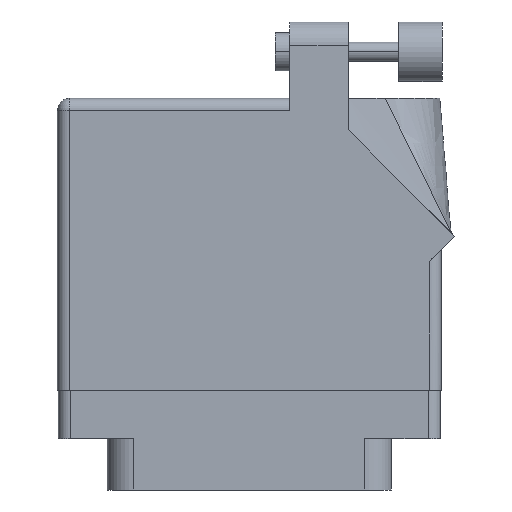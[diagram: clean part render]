
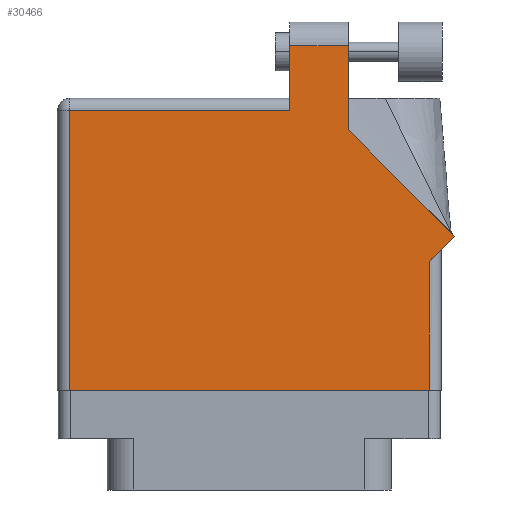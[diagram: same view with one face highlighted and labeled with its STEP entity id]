
A CAD part, front view. The second image highlights one B-rep face of the part: STEP entity #30466.
In plain terms, the highlighted face is planar.
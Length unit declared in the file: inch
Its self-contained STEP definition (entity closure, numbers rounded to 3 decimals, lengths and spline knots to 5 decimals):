
#213 = CARTESIAN_POINT ( 'NONE',  ( 0.212, 1.368, 0.455 ) ) ;
#639 = CARTESIAN_POINT ( 'NONE',  ( -0.943, 1.368, 0.455 ) ) ;
#979 = ORIENTED_EDGE ( 'NONE', *, *, #24582, .T. ) ;
#1289 = EDGE_CURVE ( 'NONE', #29988, #12275, #23878, .T. ) ;
#1784 = DIRECTION ( 'NONE',  ( -1., 0., 0. ) ) ;
#2390 = EDGE_CURVE ( 'NONE', #29772, #34692, #10206, .T. ) ;
#2638 = PLANE ( 'NONE',  #9270 ) ;
#3045 = LINE ( 'NONE', #6669, #29718 ) ;
#3461 = VECTOR ( 'NONE', #24948, 39.37008 ) ;
#4807 = LINE ( 'NONE', #32205, #32916 ) ;
#5456 = LINE ( 'NONE', #22953, #29227 ) ;
#5742 = LINE ( 'NONE', #32565, #14927 ) ;
#6669 = CARTESIAN_POINT ( 'NONE',  ( -1.005, -0.1, 0.455 ) ) ;
#8567 = ORIENTED_EDGE ( 'NONE', *, *, #14631, .T. ) ;
#9125 = DIRECTION ( 'NONE',  ( 0., 1., 0. ) ) ;
#9270 = AXIS2_PLACEMENT_3D ( 'NONE', #9371, #24231, #34086 ) ;
#9371 = CARTESIAN_POINT ( 'NONE',  ( -1.005, 1.43, 0.455 ) ) ;
#9866 = VERTEX_POINT ( 'NONE', #639 ) ;
#10206 = LINE ( 'NONE', #15218, #3461 ) ;
#11304 = LINE ( 'NONE', #17527, #31188 ) ;
#12275 = VERTEX_POINT ( 'NONE', #30609 ) ;
#13016 = ORIENTED_EDGE ( 'NONE', *, *, #13894, .T. ) ;
#13395 = DIRECTION ( 'NONE',  ( 0., -1., 0. ) ) ;
#13480 = CARTESIAN_POINT ( 'NONE',  ( 0.943, -0.1, 0.455 ) ) ;
#13894 = EDGE_CURVE ( 'NONE', #19553, #21719, #21740, .T. ) ;
#14631 = EDGE_CURVE ( 'NONE', #12275, #29772, #5742, .T. ) ;
#14927 = VECTOR ( 'NONE', #38825, 39.37008 ) ;
#15218 = CARTESIAN_POINT ( 'NONE',  ( 1.07571, 0.70771, 0.455 ) ) ;
#15445 = ORIENTED_EDGE ( 'NONE', *, *, #29038, .T. ) ;
#16708 = DIRECTION ( 'NONE',  ( -1., 0., 0. ) ) ;
#17527 = CARTESIAN_POINT ( 'NONE',  ( 0.519, 1.26442, 0.455 ) ) ;
#19553 = VERTEX_POINT ( 'NONE', #27181 ) ;
#19788 = EDGE_CURVE ( 'NONE', #34692, #29739, #11304, .T. ) ;
#20684 = LINE ( 'NONE', #25569, #35840 ) ;
#20914 = CARTESIAN_POINT ( 'NONE',  ( 1.07571, 0.70771, 0.455 ) ) ;
#21719 = VERTEX_POINT ( 'NONE', #213 ) ;
#21740 = LINE ( 'NONE', #31262, #31007 ) ;
#22588 = ORIENTED_EDGE ( 'NONE', *, *, #39192, .T. ) ;
#22953 = CARTESIAN_POINT ( 'NONE',  ( 0.212, 1.705, 0.455 ) ) ;
#23878 = LINE ( 'NONE', #39798, #24376 ) ;
#23917 = ORIENTED_EDGE ( 'NONE', *, *, #2390, .T. ) ;
#24231 = DIRECTION ( 'NONE',  ( 0., 0., -1. ) ) ;
#24376 = VECTOR ( 'NONE', #9125, 39.37008 ) ;
#24582 = EDGE_CURVE ( 'NONE', #21719, #9866, #4807, .T. ) ;
#24623 = EDGE_LOOP ( 'NONE', ( #30348, #15445, #13016, #979, #22588, #35326, #24881, #8567, #23917 ) ) ;
#24881 = ORIENTED_EDGE ( 'NONE', *, *, #1289, .T. ) ;
#24924 = DIRECTION ( 'NONE',  ( 1., 0., 0. ) ) ;
#24948 = DIRECTION ( 'NONE',  ( -0.707, 0.707, 0. ) ) ;
#25202 = FACE_OUTER_BOUND ( 'NONE', #24623, .T. ) ;
#25255 = DIRECTION ( 'NONE',  ( 0., -1., 0. ) ) ;
#25569 = CARTESIAN_POINT ( 'NONE',  ( -0.943, -0.1, 0.455 ) ) ;
#27181 = CARTESIAN_POINT ( 'NONE',  ( 0.212, 1.705, 0.455 ) ) ;
#29038 = EDGE_CURVE ( 'NONE', #29739, #19553, #5456, .T. ) ;
#29227 = VECTOR ( 'NONE', #1784, 39.37008 ) ;
#29718 = VECTOR ( 'NONE', #24924, 39.37008 ) ;
#29739 = VERTEX_POINT ( 'NONE', #30586 ) ;
#29772 = VERTEX_POINT ( 'NONE', #20914 ) ;
#29918 = CARTESIAN_POINT ( 'NONE',  ( 0.519, 1.26442, 0.455 ) ) ;
#29988 = VERTEX_POINT ( 'NONE', #13480 ) ;
#30348 = ORIENTED_EDGE ( 'NONE', *, *, #19788, .T. ) ;
#30466 = ADVANCED_FACE ( 'NONE', ( #25202 ), #2638, .F. ) ;
#30586 = CARTESIAN_POINT ( 'NONE',  ( 0.519, 1.705, 0.455 ) ) ;
#30609 = CARTESIAN_POINT ( 'NONE',  ( 0.943, 0.575, 0.455 ) ) ;
#31007 = VECTOR ( 'NONE', #25255, 39.37008 ) ;
#31188 = VECTOR ( 'NONE', #33038, 39.37008 ) ;
#31262 = CARTESIAN_POINT ( 'NONE',  ( 0.212, 1.43, 0.455 ) ) ;
#31306 = CARTESIAN_POINT ( 'NONE',  ( -0.943, -0.1, 0.455 ) ) ;
#32205 = CARTESIAN_POINT ( 'NONE',  ( -1.005, 1.368, 0.455 ) ) ;
#32500 = VERTEX_POINT ( 'NONE', #31306 ) ;
#32565 = CARTESIAN_POINT ( 'NONE',  ( 1.005, 0.637, 0.455 ) ) ;
#32916 = VECTOR ( 'NONE', #16708, 39.37008 ) ;
#33038 = DIRECTION ( 'NONE',  ( 0., 1., 0. ) ) ;
#33702 = EDGE_CURVE ( 'NONE', #32500, #29988, #3045, .T. ) ;
#34086 = DIRECTION ( 'NONE',  ( -1., 0., 0. ) ) ;
#34692 = VERTEX_POINT ( 'NONE', #29918 ) ;
#35326 = ORIENTED_EDGE ( 'NONE', *, *, #33702, .T. ) ;
#35840 = VECTOR ( 'NONE', #13395, 39.37008 ) ;
#38825 = DIRECTION ( 'NONE',  ( 0.707, 0.707, 0. ) ) ;
#39192 = EDGE_CURVE ( 'NONE', #9866, #32500, #20684, .T. ) ;
#39798 = CARTESIAN_POINT ( 'NONE',  ( 0.943, 0.637, 0.455 ) ) ;
